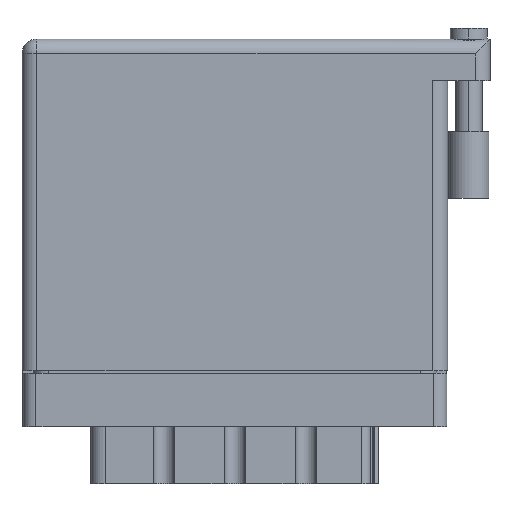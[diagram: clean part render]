
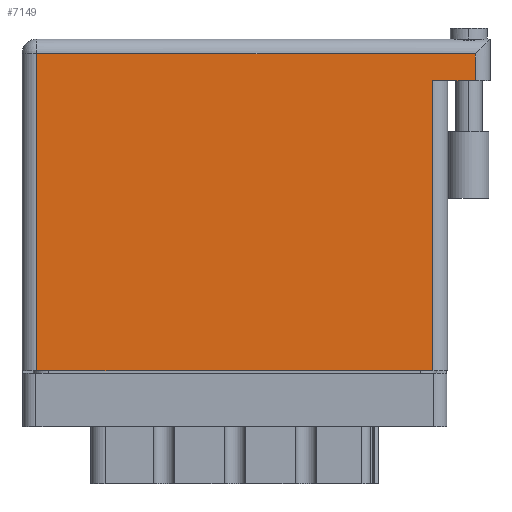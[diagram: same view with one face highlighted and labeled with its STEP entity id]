
A CAD part, front view. The second image highlights one B-rep face of the part: STEP entity #7149.
In plain terms, the highlighted face is planar.
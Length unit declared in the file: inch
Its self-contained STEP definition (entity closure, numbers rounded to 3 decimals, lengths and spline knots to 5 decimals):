
#1019 = AXIS2_PLACEMENT_3D ( 'NONE', #4903, #21193, #11662 ) ;
#2126 = CARTESIAN_POINT ( 'NONE',  ( 2.138, 1.566, 0. ) ) ;
#2540 = CARTESIAN_POINT ( 'NONE',  ( 0., 1.496, 0. ) ) ;
#2690 = CARTESIAN_POINT ( 'NONE',  ( 0., 0., 0. ) ) ;
#3209 = EDGE_CURVE ( 'NONE', #6541, #28980, #17722, .T. ) ;
#3682 = DIRECTION ( 'NONE',  ( 0., -1., 0. ) ) ;
#4469 = VERTEX_POINT ( 'NONE', #13909 ) ;
#4675 = LINE ( 'NONE', #2126, #6664 ) ;
#4903 = CARTESIAN_POINT ( 'NONE',  ( 0., 1.566, 0. ) ) ;
#5781 = VERTEX_POINT ( 'NONE', #22965 ) ;
#5807 = DIRECTION ( 'NONE',  ( 0., 1., 0. ) ) ;
#5941 = VECTOR ( 'NONE', #37195, 39.37008 ) ;
#6385 = DIRECTION ( 'NONE',  ( -1., 0., 0. ) ) ;
#6541 = VERTEX_POINT ( 'NONE', #34666 ) ;
#6664 = VECTOR ( 'NONE', #21183, 39.37008 ) ;
#7149 = ADVANCED_FACE ( 'NONE', ( #8111 ), #33840, .F. ) ;
#7373 = LINE ( 'NONE', #34502, #9833 ) ;
#7421 = ORIENTED_EDGE ( 'NONE', *, *, #29760, .T. ) ;
#8111 = FACE_OUTER_BOUND ( 'NONE', #35264, .T. ) ;
#8332 = VECTOR ( 'NONE', #5807, 39.37008 ) ;
#8872 = ORIENTED_EDGE ( 'NONE', *, *, #25938, .T. ) ;
#9833 = VECTOR ( 'NONE', #6385, 39.37008 ) ;
#10019 = CARTESIAN_POINT ( 'NONE',  ( 2.138, 1.369, 0. ) ) ;
#10986 = VERTEX_POINT ( 'NONE', #32013 ) ;
#11185 = VERTEX_POINT ( 'NONE', #10019 ) ;
#11662 = DIRECTION ( 'NONE',  ( -1., 0., 0. ) ) ;
#13909 = CARTESIAN_POINT ( 'NONE',  ( 2.138, 1.496, 0. ) ) ;
#14525 = VECTOR ( 'NONE', #3682, 39.37008 ) ;
#15219 = DIRECTION ( 'NONE',  ( -1., 0., 0. ) ) ;
#15941 = ORIENTED_EDGE ( 'NONE', *, *, #35616, .T. ) ;
#16089 = CARTESIAN_POINT ( 'NONE',  ( 0.07, 0., 0. ) ) ;
#17722 = LINE ( 'NONE', #30630, #8332 ) ;
#20447 = LINE ( 'NONE', #16089, #14525 ) ;
#21109 = ORIENTED_EDGE ( 'NONE', *, *, #3209, .T. ) ;
#21183 = DIRECTION ( 'NONE',  ( 0., 1., 0. ) ) ;
#21193 = DIRECTION ( 'NONE',  ( 0., 0., -1. ) ) ;
#21510 = LINE ( 'NONE', #2540, #30861 ) ;
#22066 = EDGE_CURVE ( 'NONE', #5781, #6541, #39977, .T. ) ;
#22965 = CARTESIAN_POINT ( 'NONE',  ( 0.07, 0., 0. ) ) ;
#25938 = EDGE_CURVE ( 'NONE', #4469, #10986, #21510, .T. ) ;
#26896 = ORIENTED_EDGE ( 'NONE', *, *, #22066, .T. ) ;
#28980 = VERTEX_POINT ( 'NONE', #35702 ) ;
#29760 = EDGE_CURVE ( 'NONE', #11185, #4469, #4675, .T. ) ;
#30630 = CARTESIAN_POINT ( 'NONE',  ( 1.938, 1.369, 0. ) ) ;
#30861 = VECTOR ( 'NONE', #15219, 39.37008 ) ;
#32013 = CARTESIAN_POINT ( 'NONE',  ( 0.07, 1.496, 0. ) ) ;
#33840 = PLANE ( 'NONE',  #1019 ) ;
#34502 = CARTESIAN_POINT ( 'NONE',  ( 2.208, 1.369, 0. ) ) ;
#34666 = CARTESIAN_POINT ( 'NONE',  ( 1.938, 0., 0. ) ) ;
#35264 = EDGE_LOOP ( 'NONE', ( #26896, #21109, #37785, #7421, #8872, #15941 ) ) ;
#35616 = EDGE_CURVE ( 'NONE', #10986, #5781, #20447, .T. ) ;
#35702 = CARTESIAN_POINT ( 'NONE',  ( 1.938, 1.369, 0. ) ) ;
#37195 = DIRECTION ( 'NONE',  ( 1., 0., 0. ) ) ;
#37785 = ORIENTED_EDGE ( 'NONE', *, *, #39323, .F. ) ;
#39323 = EDGE_CURVE ( 'NONE', #11185, #28980, #7373, .T. ) ;
#39977 = LINE ( 'NONE', #2690, #5941 ) ;
